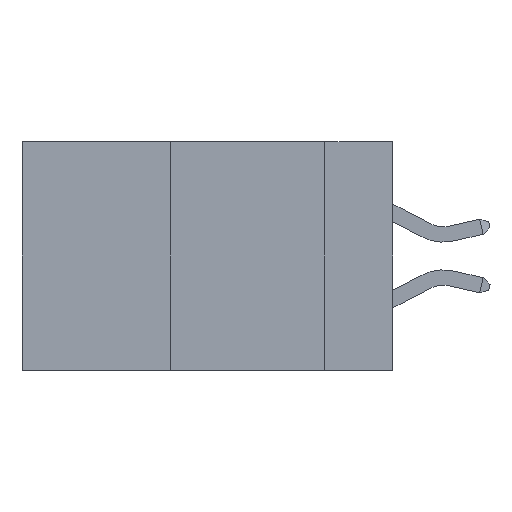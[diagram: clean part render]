
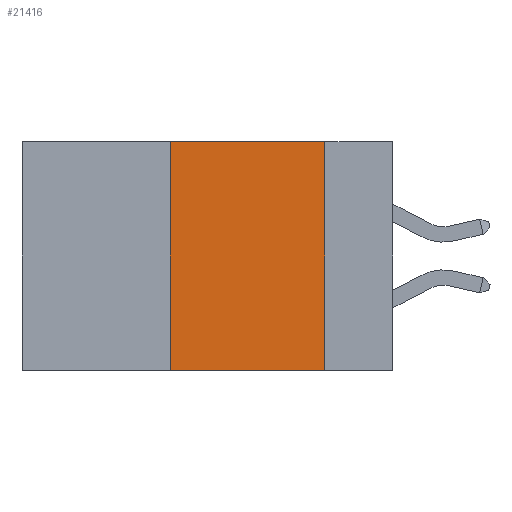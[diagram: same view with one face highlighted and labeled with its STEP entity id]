
A CAD part, left-side view. The second image highlights one B-rep face of the part: STEP entity #21416.
In plain terms, the highlighted planar face has unit normal (-1, 0, 0).
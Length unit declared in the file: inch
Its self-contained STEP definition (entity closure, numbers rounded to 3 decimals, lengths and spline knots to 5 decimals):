
#198 = DIRECTION ( 'NONE',  ( 0., 0., -1. ) ) ;
#518 = DIRECTION ( 'NONE',  ( 0., -1., 0. ) ) ;
#1284 = EDGE_CURVE ( 'NONE', #20321, #19182, #2196, .T. ) ;
#1403 = FACE_OUTER_BOUND ( 'NONE', #12555, .T. ) ;
#1415 = ORIENTED_EDGE ( 'NONE', *, *, #18204, .T. ) ;
#1531 = LINE ( 'NONE', #2923, #17786 ) ;
#2196 = LINE ( 'NONE', #9697, #9121 ) ;
#2202 = EDGE_CURVE ( 'NONE', #15595, #20321, #10460, .T. ) ;
#2923 = CARTESIAN_POINT ( 'NONE',  ( 0., 0.6, -0.37 ) ) ;
#2954 = DIRECTION ( 'NONE',  ( 0., 0., 1. ) ) ;
#2993 = EDGE_CURVE ( 'NONE', #3424, #15595, #12809, .T. ) ;
#3008 = DIRECTION ( 'NONE',  ( 0., 0., -1. ) ) ;
#3424 = VERTEX_POINT ( 'NONE', #19837 ) ;
#3626 = CARTESIAN_POINT ( 'NONE',  ( 0., 0.11, 0. ) ) ;
#6845 = CARTESIAN_POINT ( 'NONE',  ( 0., 0.6, 0. ) ) ;
#8651 = AXIS2_PLACEMENT_3D ( 'NONE', #12963, #23859, #198 ) ;
#9121 = VECTOR ( 'NONE', #3008, 39.37008 ) ;
#9697 = CARTESIAN_POINT ( 'NONE',  ( 0., 0.11, 0. ) ) ;
#9773 = VECTOR ( 'NONE', #518, 39.37008 ) ;
#10079 = VECTOR ( 'NONE', #2954, 39.37008 ) ;
#10460 = LINE ( 'NONE', #6845, #9773 ) ;
#12555 = EDGE_LOOP ( 'NONE', ( #15866, #20499, #20180, #1415 ) ) ;
#12809 = LINE ( 'NONE', #26944, #10079 ) ;
#12963 = CARTESIAN_POINT ( 'NONE',  ( 0., 0.6, 0. ) ) ;
#13059 = PLANE ( 'NONE',  #8651 ) ;
#15595 = VERTEX_POINT ( 'NONE', #23150 ) ;
#15866 = ORIENTED_EDGE ( 'NONE', *, *, #1284, .F. ) ;
#17786 = VECTOR ( 'NONE', #26729, 39.37008 ) ;
#18204 = EDGE_CURVE ( 'NONE', #3424, #19182, #1531, .T. ) ;
#18925 = CARTESIAN_POINT ( 'NONE',  ( 0., 0.11, -0.37 ) ) ;
#19182 = VERTEX_POINT ( 'NONE', #18925 ) ;
#19837 = CARTESIAN_POINT ( 'NONE',  ( 0., 0.36, -0.37 ) ) ;
#20180 = ORIENTED_EDGE ( 'NONE', *, *, #2993, .F. ) ;
#20321 = VERTEX_POINT ( 'NONE', #3626 ) ;
#20499 = ORIENTED_EDGE ( 'NONE', *, *, #2202, .F. ) ;
#21416 = ADVANCED_FACE ( 'NONE', ( #1403 ), #13059, .F. ) ;
#23150 = CARTESIAN_POINT ( 'NONE',  ( 0., 0.36, 0. ) ) ;
#23859 = DIRECTION ( 'NONE',  ( 1., 0., 0. ) ) ;
#26729 = DIRECTION ( 'NONE',  ( 0., -1., 0. ) ) ;
#26944 = CARTESIAN_POINT ( 'NONE',  ( 0., 0.36, 0. ) ) ;
